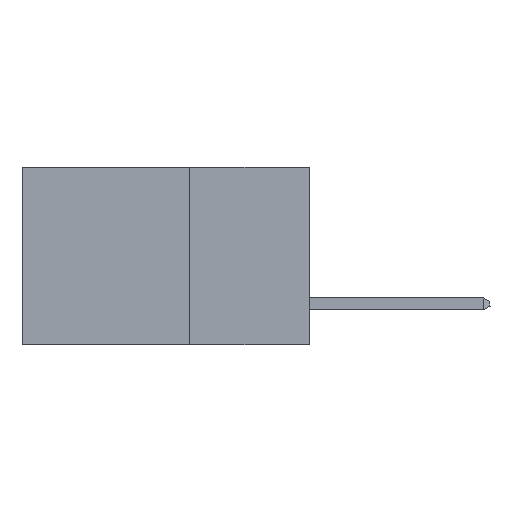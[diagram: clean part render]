
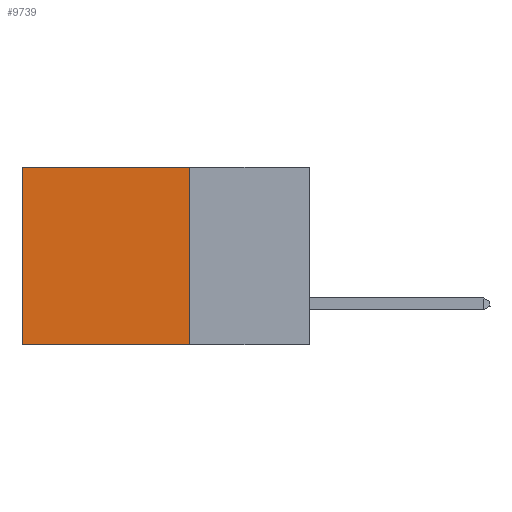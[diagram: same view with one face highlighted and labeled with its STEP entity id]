
A CAD part, left-side view. The second image highlights one B-rep face of the part: STEP entity #9739.
In plain terms, the highlighted planar face has unit normal (-1, 0, 0).
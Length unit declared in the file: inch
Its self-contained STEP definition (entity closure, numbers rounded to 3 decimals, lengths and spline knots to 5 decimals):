
#918 = CARTESIAN_POINT ( 'NONE',  ( 0.2875, 0.6, 0. ) ) ;
#2028 = EDGE_LOOP ( 'NONE', ( #8786, #9838, #5220, #5083 ) ) ;
#2495 = LINE ( 'NONE', #7413, #7044 ) ;
#2693 = VERTEX_POINT ( 'NONE', #918 ) ;
#3044 = DIRECTION ( 'NONE',  ( 1., 0., 0. ) ) ;
#3340 = DIRECTION ( 'NONE',  ( 0., 1., 0. ) ) ;
#3766 = CARTESIAN_POINT ( 'NONE',  ( 0.2875, 0.25, -0.37 ) ) ;
#3987 = VERTEX_POINT ( 'NONE', #7817 ) ;
#4201 = EDGE_CURVE ( 'NONE', #10884, #3987, #5288, .T. ) ;
#4283 = EDGE_CURVE ( 'NONE', #2693, #3987, #2495, .T. ) ;
#4355 = EDGE_CURVE ( 'NONE', #6442, #10884, #11595, .T. ) ;
#4693 = CARTESIAN_POINT ( 'NONE',  ( 0.2875, 0.25, 0. ) ) ;
#5083 = ORIENTED_EDGE ( 'NONE', *, *, #10861, .T. ) ;
#5220 = ORIENTED_EDGE ( 'NONE', *, *, #4355, .F. ) ;
#5288 = LINE ( 'NONE', #12267, #10386 ) ;
#6265 = PLANE ( 'NONE',  #11808 ) ;
#6442 = VERTEX_POINT ( 'NONE', #10475 ) ;
#6726 = DIRECTION ( 'NONE',  ( 0., 1., 0. ) ) ;
#7018 = VECTOR ( 'NONE', #6726, 39.37008 ) ;
#7044 = VECTOR ( 'NONE', #9450, 39.37008 ) ;
#7413 = CARTESIAN_POINT ( 'NONE',  ( 0.2875, 0.6, 0. ) ) ;
#7817 = CARTESIAN_POINT ( 'NONE',  ( 0.2875, 0.6, -0.37 ) ) ;
#8287 = CARTESIAN_POINT ( 'NONE',  ( 0.2875, 0.25, 0. ) ) ;
#8766 = LINE ( 'NONE', #12696, #7018 ) ;
#8786 = ORIENTED_EDGE ( 'NONE', *, *, #4283, .T. ) ;
#9339 = DIRECTION ( 'NONE',  ( 0., 0., -1. ) ) ;
#9450 = DIRECTION ( 'NONE',  ( 0., 0., -1. ) ) ;
#9636 = DIRECTION ( 'NONE',  ( 0., 0., -1. ) ) ;
#9739 = ADVANCED_FACE ( 'NONE', ( #12282 ), #6265, .F. ) ;
#9838 = ORIENTED_EDGE ( 'NONE', *, *, #4201, .F. ) ;
#10386 = VECTOR ( 'NONE', #3340, 39.37008 ) ;
#10475 = CARTESIAN_POINT ( 'NONE',  ( 0.2875, 0.25, 0. ) ) ;
#10861 = EDGE_CURVE ( 'NONE', #6442, #2693, #8766, .T. ) ;
#10884 = VERTEX_POINT ( 'NONE', #3766 ) ;
#11215 = VECTOR ( 'NONE', #9636, 39.37008 ) ;
#11595 = LINE ( 'NONE', #4693, #11215 ) ;
#11808 = AXIS2_PLACEMENT_3D ( 'NONE', #8287, #3044, #9339 ) ;
#12267 = CARTESIAN_POINT ( 'NONE',  ( 0.2875, 0.25, -0.37 ) ) ;
#12282 = FACE_OUTER_BOUND ( 'NONE', #2028, .T. ) ;
#12696 = CARTESIAN_POINT ( 'NONE',  ( 0.2875, 0.25, 0. ) ) ;
